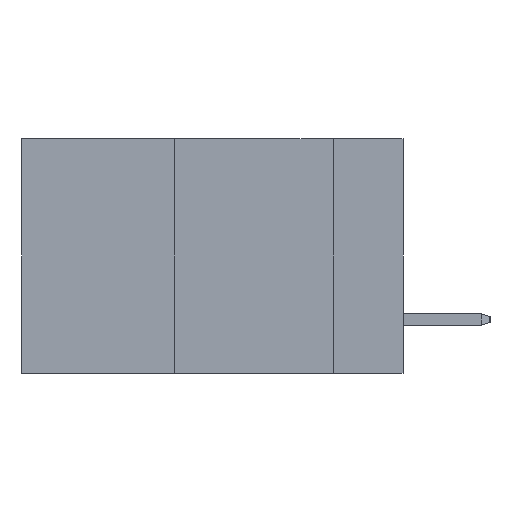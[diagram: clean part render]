
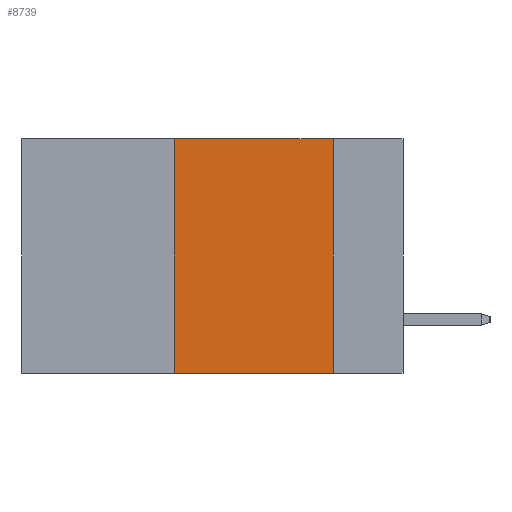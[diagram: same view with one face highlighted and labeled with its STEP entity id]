
A CAD part, left-side view. The second image highlights one B-rep face of the part: STEP entity #8739.
In plain terms, the highlighted planar face has unit normal (-1, 0, 0).
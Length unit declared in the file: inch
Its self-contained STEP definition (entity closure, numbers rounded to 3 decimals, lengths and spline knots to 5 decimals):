
#172 = ORIENTED_EDGE ( 'NONE', *, *, #11428, .F. ) ;
#410 = EDGE_CURVE ( 'NONE', #11359, #6515, #10493, .T. ) ;
#450 = DIRECTION ( 'NONE',  ( 0., 0., -1. ) ) ;
#555 = CARTESIAN_POINT ( 'NONE',  ( 0., 0.11, -0.37 ) ) ;
#2226 = ORIENTED_EDGE ( 'NONE', *, *, #410, .F. ) ;
#2574 = ORIENTED_EDGE ( 'NONE', *, *, #3075, .T. ) ;
#2887 = FACE_OUTER_BOUND ( 'NONE', #7587, .T. ) ;
#3075 = EDGE_CURVE ( 'NONE', #12354, #6515, #7102, .T. ) ;
#3330 = VECTOR ( 'NONE', #5817, 39.37008 ) ;
#3976 = DIRECTION ( 'NONE',  ( 0., -1., 0. ) ) ;
#4110 = VECTOR ( 'NONE', #450, 39.37008 ) ;
#4134 = CARTESIAN_POINT ( 'NONE',  ( 0., 0.36, 0. ) ) ;
#4346 = CARTESIAN_POINT ( 'NONE',  ( 0., 0.11, 0. ) ) ;
#4545 = CARTESIAN_POINT ( 'NONE',  ( 0., 0.36, 0. ) ) ;
#4946 = CARTESIAN_POINT ( 'NONE',  ( 0., 0.36, -0.37 ) ) ;
#4979 = CARTESIAN_POINT ( 'NONE',  ( 0., 0.6, 0. ) ) ;
#5817 = DIRECTION ( 'NONE',  ( 0., -1., 0. ) ) ;
#5848 = EDGE_CURVE ( 'NONE', #6423, #11359, #7015, .T. ) ;
#6423 = VERTEX_POINT ( 'NONE', #4134 ) ;
#6495 = ORIENTED_EDGE ( 'NONE', *, *, #5848, .F. ) ;
#6515 = VERTEX_POINT ( 'NONE', #555 ) ;
#6905 = VECTOR ( 'NONE', #12748, 39.37008 ) ;
#7015 = LINE ( 'NONE', #4979, #3330 ) ;
#7102 = LINE ( 'NONE', #8176, #7422 ) ;
#7422 = VECTOR ( 'NONE', #3976, 39.37008 ) ;
#7587 = EDGE_LOOP ( 'NONE', ( #2226, #6495, #172, #2574 ) ) ;
#7655 = LINE ( 'NONE', #4545, #6905 ) ;
#8176 = CARTESIAN_POINT ( 'NONE',  ( 0., 0.6, -0.37 ) ) ;
#8739 = ADVANCED_FACE ( 'NONE', ( #2887 ), #11915, .F. ) ;
#9535 = CARTESIAN_POINT ( 'NONE',  ( 0., 0.11, 0. ) ) ;
#9922 = DIRECTION ( 'NONE',  ( 1., 0., 0. ) ) ;
#10493 = LINE ( 'NONE', #4346, #4110 ) ;
#11061 = CARTESIAN_POINT ( 'NONE',  ( 0., 0.6, 0. ) ) ;
#11359 = VERTEX_POINT ( 'NONE', #9535 ) ;
#11428 = EDGE_CURVE ( 'NONE', #12354, #6423, #7655, .T. ) ;
#11915 = PLANE ( 'NONE',  #12859 ) ;
#12354 = VERTEX_POINT ( 'NONE', #4946 ) ;
#12748 = DIRECTION ( 'NONE',  ( 0., 0., 1. ) ) ;
#12859 = AXIS2_PLACEMENT_3D ( 'NONE', #11061, #9922, #13137 ) ;
#13137 = DIRECTION ( 'NONE',  ( 0., 0., -1. ) ) ;
